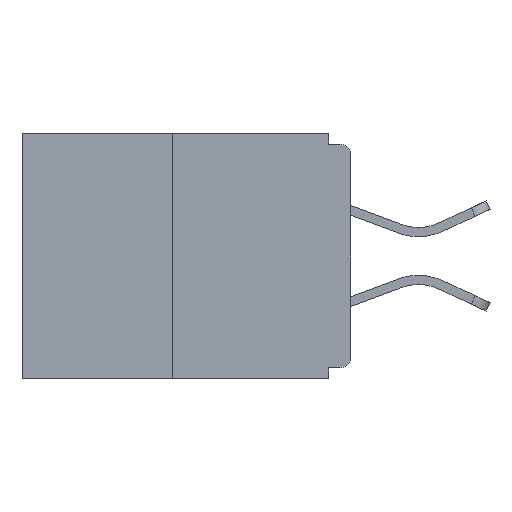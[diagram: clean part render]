
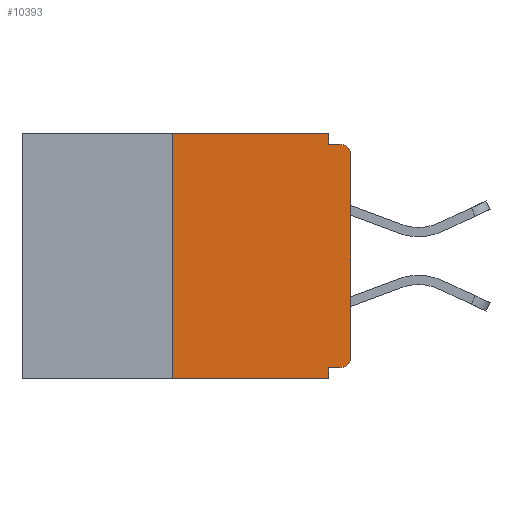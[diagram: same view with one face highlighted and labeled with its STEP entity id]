
A CAD part, left-side view. The second image highlights one B-rep face of the part: STEP entity #10393.
In plain terms, the highlighted planar face has unit normal (-1, 0, 0).
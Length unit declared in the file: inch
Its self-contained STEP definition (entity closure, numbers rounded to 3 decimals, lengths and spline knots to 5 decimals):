
#259 = ORIENTED_EDGE ( 'NONE', *, *, #18370, .F. ) ;
#999 = CARTESIAN_POINT ( 'NONE',  ( 0., 0., -0.03 ) ) ;
#1492 = PLANE ( 'NONE',  #14483 ) ;
#1542 = VECTOR ( 'NONE', #22439, 39.37008 ) ;
#1585 = DIRECTION ( 'NONE',  ( 0., 0., -1. ) ) ;
#1675 = EDGE_CURVE ( 'NONE', #20668, #8062, #21087, .T. ) ;
#1680 = CARTESIAN_POINT ( 'NONE',  ( 0., 0.25, 0. ) ) ;
#2090 = EDGE_CURVE ( 'NONE', #10899, #6185, #25155, .T. ) ;
#2525 = DIRECTION ( 'NONE',  ( 0., 0., -1. ) ) ;
#2556 = ORIENTED_EDGE ( 'NONE', *, *, #18030, .T. ) ;
#2723 = VERTEX_POINT ( 'NONE', #999 ) ;
#2990 = VECTOR ( 'NONE', #13221, 39.37008 ) ;
#3134 = LINE ( 'NONE', #18479, #1542 ) ;
#3365 = LINE ( 'NONE', #14429, #4627 ) ;
#4230 = ORIENTED_EDGE ( 'NONE', *, *, #2090, .F. ) ;
#4459 = EDGE_CURVE ( 'NONE', #25367, #20825, #7073, .T. ) ;
#4627 = VECTOR ( 'NONE', #6478, 39.37008 ) ;
#5034 = CARTESIAN_POINT ( 'NONE',  ( 0., 0.25, -0.343 ) ) ;
#5917 = AXIS2_PLACEMENT_3D ( 'NONE', #25801, #21831, #24037 ) ;
#6163 = EDGE_CURVE ( 'NONE', #25367, #6185, #12680, .T. ) ;
#6185 = VERTEX_POINT ( 'NONE', #8156 ) ;
#6478 = DIRECTION ( 'NONE',  ( 0., -1., 0. ) ) ;
#7073 = LINE ( 'NONE', #1680, #19566 ) ;
#7201 = CARTESIAN_POINT ( 'NONE',  ( 0., 0.031, -0.343 ) ) ;
#7518 = DIRECTION ( 'NONE',  ( 0., 0., 1. ) ) ;
#7702 = VERTEX_POINT ( 'NONE', #20703 ) ;
#7897 = DIRECTION ( 'NONE',  ( 0., -1., 0. ) ) ;
#8062 = VERTEX_POINT ( 'NONE', #22671 ) ;
#8156 = CARTESIAN_POINT ( 'NONE',  ( 0., 0.031, -0.343 ) ) ;
#8266 = ORIENTED_EDGE ( 'NONE', *, *, #12142, .F. ) ;
#8347 = CARTESIAN_POINT ( 'NONE',  ( 0., 0.031, 0. ) ) ;
#10188 = AXIS2_PLACEMENT_3D ( 'NONE', #14017, #10286, #20019 ) ;
#10286 = DIRECTION ( 'NONE',  ( -1., 0., 0. ) ) ;
#10393 = ADVANCED_FACE ( 'NONE', ( #21545 ), #1492, .F. ) ;
#10541 = VECTOR ( 'NONE', #2525, 39.37008 ) ;
#10899 = VERTEX_POINT ( 'NONE', #17839 ) ;
#11541 = EDGE_CURVE ( 'NONE', #20825, #14586, #3365, .T. ) ;
#11811 = CARTESIAN_POINT ( 'NONE',  ( 0., 0., -0.328 ) ) ;
#11869 = LINE ( 'NONE', #13338, #12492 ) ;
#12142 = EDGE_CURVE ( 'NONE', #20668, #10899, #19214, .T. ) ;
#12166 = CARTESIAN_POINT ( 'NONE',  ( 0., 0.46, -0.343 ) ) ;
#12241 = CARTESIAN_POINT ( 'NONE',  ( 0., 0.015, -0.015 ) ) ;
#12445 = EDGE_CURVE ( 'NONE', #14586, #7702, #21731, .T. ) ;
#12465 = CARTESIAN_POINT ( 'NONE',  ( 0., 0.031, 0. ) ) ;
#12492 = VECTOR ( 'NONE', #23133, 39.37008 ) ;
#12680 = LINE ( 'NONE', #12166, #13933 ) ;
#13221 = DIRECTION ( 'NONE',  ( 0., 0., -1. ) ) ;
#13309 = CARTESIAN_POINT ( 'NONE',  ( 0., 0.015, -0.328 ) ) ;
#13338 = CARTESIAN_POINT ( 'NONE',  ( 0., 0., -0.015 ) ) ;
#13933 = VECTOR ( 'NONE', #7897, 39.37008 ) ;
#14017 = CARTESIAN_POINT ( 'NONE',  ( 0., 0.015, -0.313 ) ) ;
#14429 = CARTESIAN_POINT ( 'NONE',  ( 0., 0.46, 0. ) ) ;
#14483 = AXIS2_PLACEMENT_3D ( 'NONE', #17445, #19528, #1585 ) ;
#14586 = VERTEX_POINT ( 'NONE', #8347 ) ;
#15033 = ORIENTED_EDGE ( 'NONE', *, *, #11541, .F. ) ;
#16550 = VERTEX_POINT ( 'NONE', #12241 ) ;
#17445 = CARTESIAN_POINT ( 'NONE',  ( 0., 0.46, 0. ) ) ;
#17672 = VECTOR ( 'NONE', #23689, 39.37008 ) ;
#17839 = CARTESIAN_POINT ( 'NONE',  ( 0., 0.031, -0.328 ) ) ;
#17860 = CARTESIAN_POINT ( 'NONE',  ( 0., 0.25, 0. ) ) ;
#18030 = EDGE_CURVE ( 'NONE', #8062, #2723, #3134, .T. ) ;
#18051 = CIRCLE ( 'NONE', #5917, 0.015 ) ;
#18370 = EDGE_CURVE ( 'NONE', #7702, #16550, #11869, .T. ) ;
#18443 = ORIENTED_EDGE ( 'NONE', *, *, #6163, .T. ) ;
#18479 = CARTESIAN_POINT ( 'NONE',  ( 0., 0., 0. ) ) ;
#18742 = EDGE_CURVE ( 'NONE', #2723, #16550, #18051, .T. ) ;
#18937 = ORIENTED_EDGE ( 'NONE', *, *, #1675, .T. ) ;
#19214 = LINE ( 'NONE', #11811, #17672 ) ;
#19528 = DIRECTION ( 'NONE',  ( 1., 0., 0. ) ) ;
#19566 = VECTOR ( 'NONE', #7518, 39.37008 ) ;
#20019 = DIRECTION ( 'NONE',  ( 0., 0., -1. ) ) ;
#20668 = VERTEX_POINT ( 'NONE', #13309 ) ;
#20703 = CARTESIAN_POINT ( 'NONE',  ( 0., 0.031, -0.015 ) ) ;
#20825 = VERTEX_POINT ( 'NONE', #17860 ) ;
#21087 = CIRCLE ( 'NONE', #10188, 0.015 ) ;
#21545 = FACE_OUTER_BOUND ( 'NONE', #22550, .T. ) ;
#21731 = LINE ( 'NONE', #12465, #10541 ) ;
#21831 = DIRECTION ( 'NONE',  ( -1., 0., 0. ) ) ;
#22439 = DIRECTION ( 'NONE',  ( 0., 0., 1. ) ) ;
#22550 = EDGE_LOOP ( 'NONE', ( #15033, #23941, #18443, #4230, #8266, #18937, #2556, #24888, #259, #25013 ) ) ;
#22671 = CARTESIAN_POINT ( 'NONE',  ( 0., 0., -0.313 ) ) ;
#23133 = DIRECTION ( 'NONE',  ( 0., -1., 0. ) ) ;
#23689 = DIRECTION ( 'NONE',  ( 0., 1., 0. ) ) ;
#23941 = ORIENTED_EDGE ( 'NONE', *, *, #4459, .F. ) ;
#24037 = DIRECTION ( 'NONE',  ( 0., 0., -1. ) ) ;
#24888 = ORIENTED_EDGE ( 'NONE', *, *, #18742, .T. ) ;
#25013 = ORIENTED_EDGE ( 'NONE', *, *, #12445, .F. ) ;
#25155 = LINE ( 'NONE', #7201, #2990 ) ;
#25367 = VERTEX_POINT ( 'NONE', #5034 ) ;
#25801 = CARTESIAN_POINT ( 'NONE',  ( 0., 0.015, -0.03 ) ) ;
